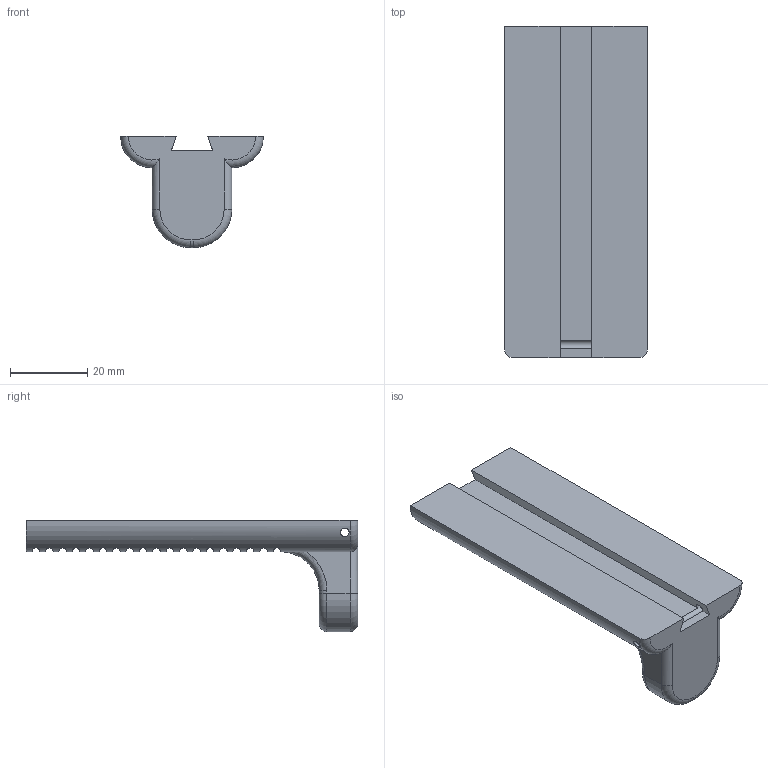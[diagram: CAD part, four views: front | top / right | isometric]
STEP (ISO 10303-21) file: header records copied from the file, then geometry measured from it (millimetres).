
FILE_DESCRIPTION(/* description */ (''),/* implementation_level */ '2;1');
FILE_NAME(/* name */ 'Shorty Handstop v10.step',/* time_stamp */ '2020-06-28T23:17:43-04:00',/* author */ (''),/* organization */ (''),/* preprocessor_version */ 'ST-DEVELOPER v18.1',/* originating_system */ 'Autodesk Translation Framework v9.3.0.1241',/* authorisation */ '');
FILE_SCHEMA (('AUTOMOTIVE_DESIGN { 1 0 10303 214 3 1 1 }'));
Length unit declared in the file: millimetre
Products named in the file (1): Shorty Handstop
Bounding box: 37 x 86 x 28.9 mm (x, y, z)
Volume: 23823.2 mm3; surface area: 10170.7 mm2
Topology: 1 solids, 1 shells, 90 faces, 258 edges, 168 vertices
Faces by surface type: cylinder 49, plane 33, torus 8
Full cylindrical faces by diameter (mm): 2.25 x1
Entity records: 3865 total; most frequent: CARTESIAN_POINT 1609, ORIENTED_EDGE 516, DIRECTION 390, EDGE_CURVE 258, VERTEX_POINT 168, LINE 140, VECTOR 140, AXIS2_PLACEMENT_3D 125
